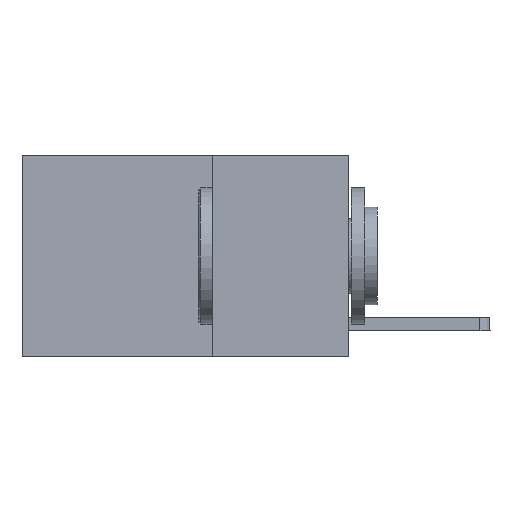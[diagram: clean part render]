
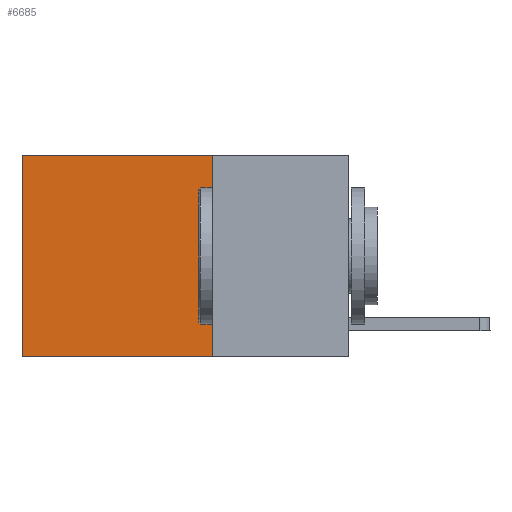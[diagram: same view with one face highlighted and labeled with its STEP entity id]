
A CAD part, left-side view. The second image highlights one B-rep face of the part: STEP entity #6685.
In plain terms, the highlighted planar face has unit normal (-1, 0, 0).
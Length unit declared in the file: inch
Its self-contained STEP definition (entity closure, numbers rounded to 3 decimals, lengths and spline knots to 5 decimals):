
#222 = CARTESIAN_POINT ( 'NONE',  ( 0.2625, 0.25, 0. ) ) ;
#843 = VECTOR ( 'NONE', #9771, 39.37008 ) ;
#989 = DIRECTION ( 'NONE',  ( 0., 1., 0. ) ) ;
#1114 = FACE_OUTER_BOUND ( 'NONE', #7462, .T. ) ;
#1442 = ORIENTED_EDGE ( 'NONE', *, *, #6764, .T. ) ;
#2061 = LINE ( 'NONE', #4846, #9160 ) ;
#2099 = DIRECTION ( 'NONE',  ( 1., 0., 0. ) ) ;
#2332 = ORIENTED_EDGE ( 'NONE', *, *, #3762, .T. ) ;
#2691 = VECTOR ( 'NONE', #8872, 39.37008 ) ;
#3003 = LINE ( 'NONE', #6714, #8052 ) ;
#3762 = EDGE_CURVE ( 'NONE', #6516, #6202, #3003, .T. ) ;
#3858 = EDGE_CURVE ( 'NONE', #9676, #6568, #7934, .T. ) ;
#4846 = CARTESIAN_POINT ( 'NONE',  ( 0.2625, 0.25, 0. ) ) ;
#5140 = CARTESIAN_POINT ( 'NONE',  ( 0.2625, 0.25, -0.37 ) ) ;
#5510 = CARTESIAN_POINT ( 'NONE',  ( 0.2625, 0.6, 0. ) ) ;
#5807 = DIRECTION ( 'NONE',  ( 0., 0., -1. ) ) ;
#6202 = VERTEX_POINT ( 'NONE', #5510 ) ;
#6516 = VERTEX_POINT ( 'NONE', #10163 ) ;
#6568 = VERTEX_POINT ( 'NONE', #10409 ) ;
#6629 = AXIS2_PLACEMENT_3D ( 'NONE', #222, #2099, #5807 ) ;
#6685 = ADVANCED_FACE ( 'NONE', ( #1114 ), #8565, .F. ) ;
#6714 = CARTESIAN_POINT ( 'NONE',  ( 0.2625, 0.25, 0. ) ) ;
#6764 = EDGE_CURVE ( 'NONE', #6202, #6568, #7838, .T. ) ;
#7462 = EDGE_LOOP ( 'NONE', ( #1442, #8319, #8195, #2332 ) ) ;
#7838 = LINE ( 'NONE', #11580, #2691 ) ;
#7934 = LINE ( 'NONE', #8728, #843 ) ;
#8052 = VECTOR ( 'NONE', #989, 39.37008 ) ;
#8195 = ORIENTED_EDGE ( 'NONE', *, *, #10882, .F. ) ;
#8319 = ORIENTED_EDGE ( 'NONE', *, *, #3858, .F. ) ;
#8565 = PLANE ( 'NONE',  #6629 ) ;
#8728 = CARTESIAN_POINT ( 'NONE',  ( 0.2625, 0.25, -0.37 ) ) ;
#8872 = DIRECTION ( 'NONE',  ( 0., 0., -1. ) ) ;
#9160 = VECTOR ( 'NONE', #10540, 39.37008 ) ;
#9676 = VERTEX_POINT ( 'NONE', #5140 ) ;
#9771 = DIRECTION ( 'NONE',  ( 0., 1., 0. ) ) ;
#10163 = CARTESIAN_POINT ( 'NONE',  ( 0.2625, 0.25, 0. ) ) ;
#10409 = CARTESIAN_POINT ( 'NONE',  ( 0.2625, 0.6, -0.37 ) ) ;
#10540 = DIRECTION ( 'NONE',  ( 0., 0., -1. ) ) ;
#10882 = EDGE_CURVE ( 'NONE', #6516, #9676, #2061, .T. ) ;
#11580 = CARTESIAN_POINT ( 'NONE',  ( 0.2625, 0.6, 0. ) ) ;
